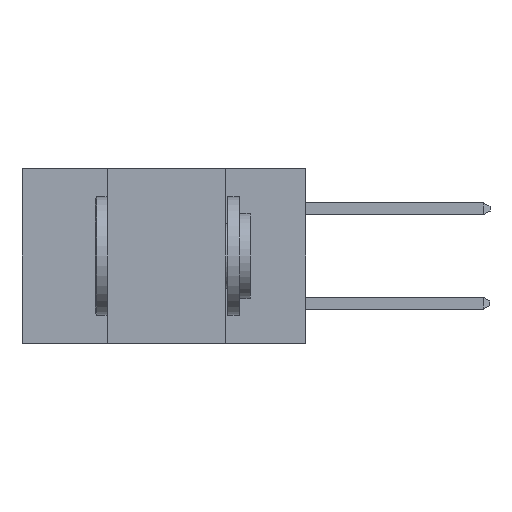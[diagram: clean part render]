
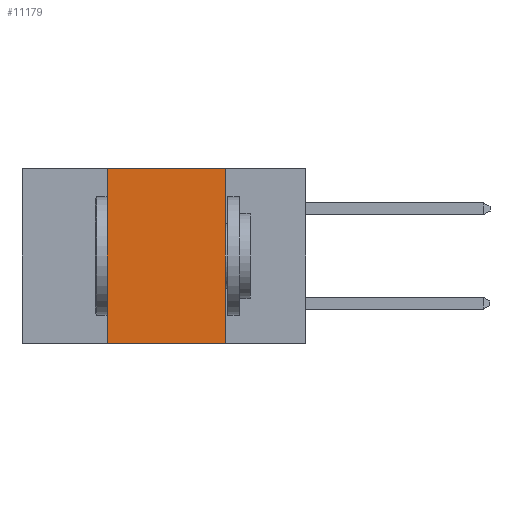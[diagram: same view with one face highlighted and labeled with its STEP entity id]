
A CAD part, left-side view. The second image highlights one B-rep face of the part: STEP entity #11179.
In plain terms, the highlighted planar face has unit normal (-1, 0, 0).
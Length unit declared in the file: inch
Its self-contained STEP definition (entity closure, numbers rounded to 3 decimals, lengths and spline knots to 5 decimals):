
#337 = EDGE_LOOP ( 'NONE', ( #28251, #11676, #6314, #19080 ) ) ;
#439 = CARTESIAN_POINT ( 'NONE',  ( 0., 0.42, 0. ) ) ;
#1156 = VECTOR ( 'NONE', #7518, 39.37008 ) ;
#2718 = DIRECTION ( 'NONE',  ( 0., 0., -1. ) ) ;
#3290 = FACE_OUTER_BOUND ( 'NONE', #337, .T. ) ;
#3869 = VECTOR ( 'NONE', #10601, 39.37008 ) ;
#4375 = VERTEX_POINT ( 'NONE', #11470 ) ;
#4653 = CARTESIAN_POINT ( 'NONE',  ( 0., 0.17, 0. ) ) ;
#4726 = CARTESIAN_POINT ( 'NONE',  ( 0., 0.6, -0.37 ) ) ;
#6314 = ORIENTED_EDGE ( 'NONE', *, *, #28826, .F. ) ;
#7026 = DIRECTION ( 'NONE',  ( 0., 0., -1. ) ) ;
#7518 = DIRECTION ( 'NONE',  ( 0., 0., 1. ) ) ;
#7594 = AXIS2_PLACEMENT_3D ( 'NONE', #23096, #16408, #2718 ) ;
#7669 = CARTESIAN_POINT ( 'NONE',  ( 0., 0.42, 0. ) ) ;
#8363 = VERTEX_POINT ( 'NONE', #13159 ) ;
#8543 = VECTOR ( 'NONE', #22772, 39.37008 ) ;
#8564 = EDGE_CURVE ( 'NONE', #8363, #13399, #26525, .T. ) ;
#10601 = DIRECTION ( 'NONE',  ( 0., -1., 0. ) ) ;
#11179 = ADVANCED_FACE ( 'NONE', ( #3290 ), #14152, .F. ) ;
#11470 = CARTESIAN_POINT ( 'NONE',  ( 0., 0.17, 0. ) ) ;
#11543 = LINE ( 'NONE', #4653, #16110 ) ;
#11676 = ORIENTED_EDGE ( 'NONE', *, *, #21370, .F. ) ;
#13159 = CARTESIAN_POINT ( 'NONE',  ( 0., 0.42, -0.37 ) ) ;
#13399 = VERTEX_POINT ( 'NONE', #15124 ) ;
#14152 = PLANE ( 'NONE',  #7594 ) ;
#15038 = CARTESIAN_POINT ( 'NONE',  ( 0., 0.6, 0. ) ) ;
#15124 = CARTESIAN_POINT ( 'NONE',  ( 0., 0.17, -0.37 ) ) ;
#16013 = LINE ( 'NONE', #15038, #3869 ) ;
#16110 = VECTOR ( 'NONE', #7026, 39.37008 ) ;
#16408 = DIRECTION ( 'NONE',  ( 1., 0., 0. ) ) ;
#17988 = VERTEX_POINT ( 'NONE', #7669 ) ;
#19080 = ORIENTED_EDGE ( 'NONE', *, *, #8564, .T. ) ;
#21370 = EDGE_CURVE ( 'NONE', #17988, #4375, #16013, .T. ) ;
#22772 = DIRECTION ( 'NONE',  ( 0., -1., 0. ) ) ;
#23096 = CARTESIAN_POINT ( 'NONE',  ( 0., 0.6, 0. ) ) ;
#23269 = LINE ( 'NONE', #439, #1156 ) ;
#24274 = EDGE_CURVE ( 'NONE', #4375, #13399, #11543, .T. ) ;
#26525 = LINE ( 'NONE', #4726, #8543 ) ;
#28251 = ORIENTED_EDGE ( 'NONE', *, *, #24274, .F. ) ;
#28826 = EDGE_CURVE ( 'NONE', #8363, #17988, #23269, .T. ) ;
